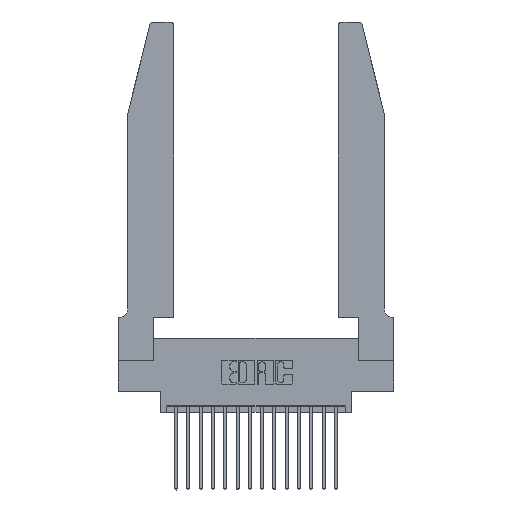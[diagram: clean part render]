
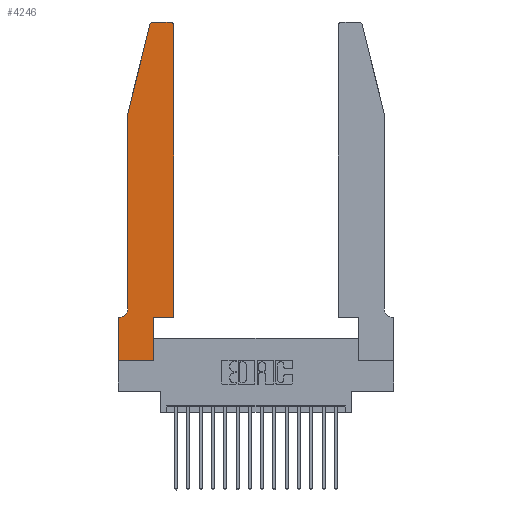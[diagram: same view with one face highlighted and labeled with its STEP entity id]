
A CAD part, top view. The second image highlights one B-rep face of the part: STEP entity #4246.
In plain terms, the highlighted planar face has unit normal (0, 0, 1).
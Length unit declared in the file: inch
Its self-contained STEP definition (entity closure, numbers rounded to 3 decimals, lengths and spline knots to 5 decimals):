
#55 = ORIENTED_EDGE ( 'NONE', *, *, #220, .T. ) ;
#194 = CARTESIAN_POINT ( 'NONE',  ( 0., 0.35, 0.37 ) ) ;
#220 = EDGE_CURVE ( 'NONE', #4896, #10859, #2325, .T. ) ;
#680 = CARTESIAN_POINT ( 'NONE',  ( 0.0055, 0.42, 0.37 ) ) ;
#1116 = CARTESIAN_POINT ( 'NONE',  ( 0.0755, 0.42, 0.37 ) ) ;
#1382 = DIRECTION ( 'NONE',  ( -0.239, -0.971, 0. ) ) ;
#1540 = CARTESIAN_POINT ( 'NONE',  ( 0.0755, 2., 0.37 ) ) ;
#1598 = EDGE_CURVE ( 'NONE', #11159, #11517, #1799, .T. ) ;
#1742 = EDGE_CURVE ( 'NONE', #4464, #18931, #2981, .T. ) ;
#1747 = CARTESIAN_POINT ( 'NONE',  ( 0.4205, 2.72, 0.37 ) ) ;
#1799 = LINE ( 'NONE', #8260, #17488 ) ;
#2044 = DIRECTION ( 'NONE',  ( 1., 0., 0. ) ) ;
#2325 = CIRCLE ( 'NONE', #16165, 0.03 ) ;
#2508 = VECTOR ( 'NONE', #17719, 39.37008 ) ;
#2981 = LINE ( 'NONE', #7083, #2508 ) ;
#4019 = CARTESIAN_POINT ( 'NONE',  ( 0., 0., 0.37 ) ) ;
#4193 = LINE ( 'NONE', #4019, #11098 ) ;
#4246 = ADVANCED_FACE ( 'NONE', ( #5049 ), #4654, .T. ) ;
#4464 = VERTEX_POINT ( 'NONE', #17735 ) ;
#4525 = DIRECTION ( 'NONE',  ( 1., 0., 0. ) ) ;
#4654 = PLANE ( 'NONE',  #6759 ) ;
#4896 = VERTEX_POINT ( 'NONE', #14277 ) ;
#5049 = FACE_OUTER_BOUND ( 'NONE', #10537, .T. ) ;
#5094 = VECTOR ( 'NONE', #11909, 39.37008 ) ;
#5109 = CARTESIAN_POINT ( 'NONE',  ( 0.284, 2.75, 0.37 ) ) ;
#5451 = CARTESIAN_POINT ( 'NONE',  ( 0.2865, 0.35, 0.37 ) ) ;
#5502 = ORIENTED_EDGE ( 'NONE', *, *, #13152, .T. ) ;
#5781 = EDGE_CURVE ( 'NONE', #10859, #9885, #15676, .T. ) ;
#6235 = AXIS2_PLACEMENT_3D ( 'NONE', #14751, #8469, #11630 ) ;
#6588 = ORIENTED_EDGE ( 'NONE', *, *, #17175, .T. ) ;
#6630 = ORIENTED_EDGE ( 'NONE', *, *, #19509, .T. ) ;
#6759 = AXIS2_PLACEMENT_3D ( 'NONE', #194, #15214, #4525 ) ;
#6949 = DIRECTION ( 'NONE',  ( 1., 0., 0. ) ) ;
#7057 = ORIENTED_EDGE ( 'NONE', *, *, #5781, .T. ) ;
#7083 = CARTESIAN_POINT ( 'NONE',  ( 0.0755, 0.35, 0.37 ) ) ;
#7116 = CARTESIAN_POINT ( 'NONE',  ( 0., 0., 0.37 ) ) ;
#7250 = CARTESIAN_POINT ( 'NONE',  ( 0.4505, 0.35, 0.37 ) ) ;
#7419 = CARTESIAN_POINT ( 'NONE',  ( 0.0755, 2., 0.37 ) ) ;
#8068 = ORIENTED_EDGE ( 'NONE', *, *, #1742, .T. ) ;
#8260 = CARTESIAN_POINT ( 'NONE',  ( 0.4505, 0.35, 0.37 ) ) ;
#8346 = CARTESIAN_POINT ( 'NONE',  ( 0.0755, 2., 0.37 ) ) ;
#8469 = DIRECTION ( 'NONE',  ( 0., 0., 1. ) ) ;
#8903 = CARTESIAN_POINT ( 'NONE',  ( 0.25487, 2.72718, 0.37 ) ) ;
#9099 = DIRECTION ( 'NONE',  ( 0., 0., 1. ) ) ;
#9115 = EDGE_CURVE ( 'NONE', #14193, #4464, #19269, .T. ) ;
#9162 = DIRECTION ( 'NONE',  ( 1., 0., 0. ) ) ;
#9229 = EDGE_CURVE ( 'NONE', #15079, #11159, #14534, .T. ) ;
#9239 = VECTOR ( 'NONE', #15207, 39.37008 ) ;
#9885 = VERTEX_POINT ( 'NONE', #5109 ) ;
#10021 = ORIENTED_EDGE ( 'NONE', *, *, #15932, .T. ) ;
#10372 = CARTESIAN_POINT ( 'NONE',  ( 0.4505, 0.35, 0.37 ) ) ;
#10511 = CARTESIAN_POINT ( 'NONE',  ( 0.2865, 0., 0.37 ) ) ;
#10537 = EDGE_LOOP ( 'NONE', ( #7057, #12806, #6630, #14803, #12985, #8068, #5502, #10021, #17605, #17336, #6588, #55 ) ) ;
#10859 = VERTEX_POINT ( 'NONE', #11313 ) ;
#11030 = VERTEX_POINT ( 'NONE', #7116 ) ;
#11047 = DIRECTION ( 'NONE',  ( -1., 0., 0. ) ) ;
#11098 = VECTOR ( 'NONE', #6949, 39.37008 ) ;
#11159 = VERTEX_POINT ( 'NONE', #12189 ) ;
#11313 = CARTESIAN_POINT ( 'NONE',  ( 0.4205, 2.75, 0.37 ) ) ;
#11472 = VECTOR ( 'NONE', #1382, 39.37008 ) ;
#11517 = VERTEX_POINT ( 'NONE', #7250 ) ;
#11630 = DIRECTION ( 'NONE',  ( 1., 0., 0. ) ) ;
#11909 = DIRECTION ( 'NONE',  ( 0., 1., 0. ) ) ;
#12189 = CARTESIAN_POINT ( 'NONE',  ( 0.2865, 0.35, 0.37 ) ) ;
#12309 = CARTESIAN_POINT ( 'NONE',  ( 0., 0.35, 0.37 ) ) ;
#12735 = VERTEX_POINT ( 'NONE', #8903 ) ;
#12806 = ORIENTED_EDGE ( 'NONE', *, *, #14188, .T. ) ;
#12914 = EDGE_CURVE ( 'NONE', #13141, #14193, #15351, .T. ) ;
#12985 = ORIENTED_EDGE ( 'NONE', *, *, #9115, .T. ) ;
#13141 = VERTEX_POINT ( 'NONE', #8346 ) ;
#13152 = EDGE_CURVE ( 'NONE', #18931, #11030, #15104, .T. ) ;
#13345 = VECTOR ( 'NONE', #19123, 39.37008 ) ;
#14188 = EDGE_CURVE ( 'NONE', #9885, #12735, #17351, .T. ) ;
#14193 = VERTEX_POINT ( 'NONE', #1116 ) ;
#14277 = CARTESIAN_POINT ( 'NONE',  ( 0.4505, 2.72, 0.37 ) ) ;
#14422 = VECTOR ( 'NONE', #16619, 39.37008 ) ;
#14534 = LINE ( 'NONE', #5451, #13345 ) ;
#14735 = AXIS2_PLACEMENT_3D ( 'NONE', #680, #15747, #11047 ) ;
#14751 = CARTESIAN_POINT ( 'NONE',  ( 0.284, 2.72, 0.37 ) ) ;
#14803 = ORIENTED_EDGE ( 'NONE', *, *, #12914, .T. ) ;
#15067 = CARTESIAN_POINT ( 'NONE',  ( 0.2605, 2.75, 0.37 ) ) ;
#15079 = VERTEX_POINT ( 'NONE', #10511 ) ;
#15104 = LINE ( 'NONE', #17350, #16304 ) ;
#15207 = DIRECTION ( 'NONE',  ( -1., 0., 0. ) ) ;
#15214 = DIRECTION ( 'NONE',  ( 0., 0., 1. ) ) ;
#15351 = LINE ( 'NONE', #1540, #14422 ) ;
#15503 = LINE ( 'NONE', #7419, #11472 ) ;
#15676 = LINE ( 'NONE', #15067, #9239 ) ;
#15747 = DIRECTION ( 'NONE',  ( 0., 0., -1. ) ) ;
#15932 = EDGE_CURVE ( 'NONE', #11030, #15079, #4193, .T. ) ;
#16165 = AXIS2_PLACEMENT_3D ( 'NONE', #1747, #9099, #9162 ) ;
#16304 = VECTOR ( 'NONE', #19053, 39.37008 ) ;
#16619 = DIRECTION ( 'NONE',  ( 0., -1., 0. ) ) ;
#17175 = EDGE_CURVE ( 'NONE', #11517, #4896, #18158, .T. ) ;
#17336 = ORIENTED_EDGE ( 'NONE', *, *, #1598, .T. ) ;
#17350 = CARTESIAN_POINT ( 'NONE',  ( 0., 0., 0.37 ) ) ;
#17351 = CIRCLE ( 'NONE', #6235, 0.03 ) ;
#17488 = VECTOR ( 'NONE', #2044, 39.37008 ) ;
#17605 = ORIENTED_EDGE ( 'NONE', *, *, #9229, .T. ) ;
#17719 = DIRECTION ( 'NONE',  ( -1., 0., 0. ) ) ;
#17735 = CARTESIAN_POINT ( 'NONE',  ( 0.0055, 0.35, 0.37 ) ) ;
#18158 = LINE ( 'NONE', #10372, #5094 ) ;
#18931 = VERTEX_POINT ( 'NONE', #12309 ) ;
#19053 = DIRECTION ( 'NONE',  ( 0., -1., 0. ) ) ;
#19123 = DIRECTION ( 'NONE',  ( 0., 1., 0. ) ) ;
#19269 = CIRCLE ( 'NONE', #14735, 0.07 ) ;
#19509 = EDGE_CURVE ( 'NONE', #12735, #13141, #15503, .T. ) ;
